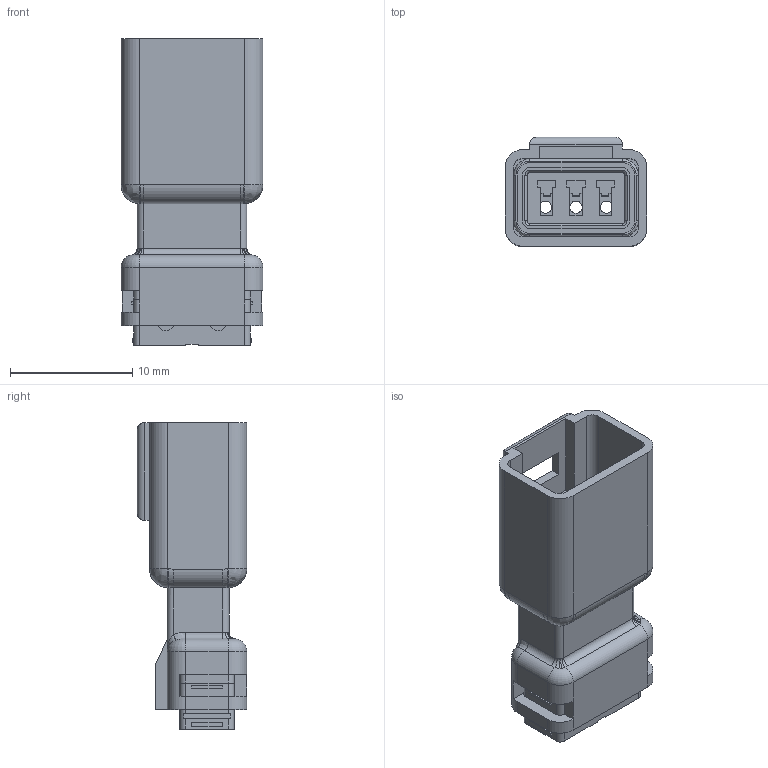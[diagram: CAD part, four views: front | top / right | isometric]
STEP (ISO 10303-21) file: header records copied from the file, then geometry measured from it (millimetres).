
FILE_DESCRIPTION (( 'STEP AP214' ), '1' );
FILE_NAME ('565-003-000-310.STEP', '2020-07-27T15:10:10', ( '' ), ( '' ), 'SwSTEP 2.0', 'SolidWorks 2020', '' );
FILE_SCHEMA (( 'AUTOMOTIVE_DESIGN' ));
Length unit declared in the file: millimetre
Products named in the file (5): 565-003-000-310; 565-003-000-310_Housing; 565-003-000-310_Rear Gasket; 565-003-000-310_Front Gasket; 565-003-000-310_Rear Insulator
Assembly tree (4 placements, depth 2):
  565-003-000-310
    565-003-000-310_Housing
    565-003-000-310_Rear Insulator
    565-003-000-310_Rear Gasket
    565-003-000-310_Front Gasket
Bounding box: 11.6 x 8.95 x 25.1 mm (x, y, z)
Volume: 1134.8 mm3; surface area: 2547 mm2
Topology: 4 solids, 4 shells, 496 faces, 1311 edges, 846 vertices
Faces by surface type: plane 259, cylinder 148, bspline 46, torus 43
Entity records: 16973 total; most frequent: CARTESIAN_POINT 4497, ORIENTED_EDGE 2614, DIRECTION 2516, EDGE_CURVE 1307, AXIS2_PLACEMENT_3D 853, VERTEX_POINT 846, LINE 810, VECTOR 810
